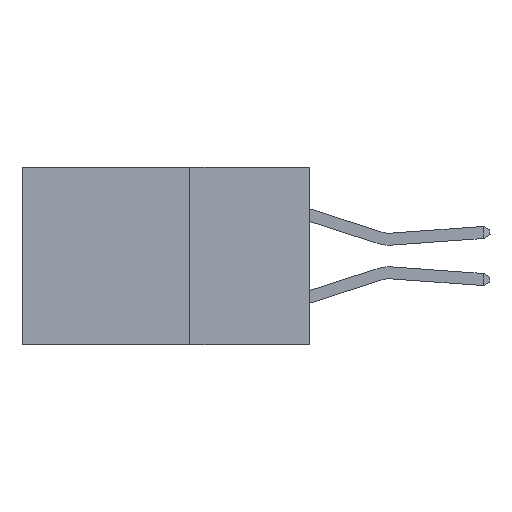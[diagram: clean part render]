
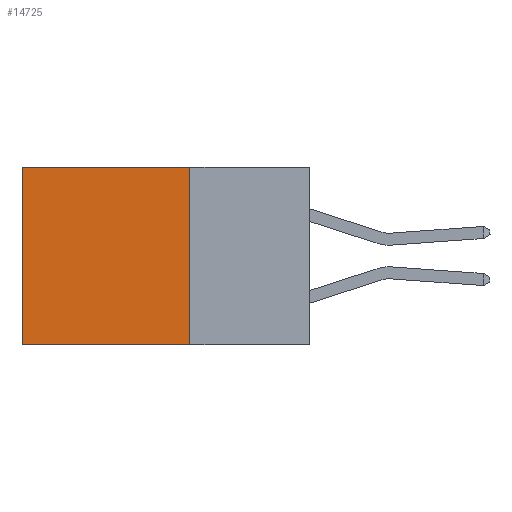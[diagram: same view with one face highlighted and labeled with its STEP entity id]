
A CAD part, left-side view. The second image highlights one B-rep face of the part: STEP entity #14725.
In plain terms, the highlighted planar face has unit normal (-1, 0, 0).
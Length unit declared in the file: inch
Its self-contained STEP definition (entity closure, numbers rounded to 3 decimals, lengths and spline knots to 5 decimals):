
#512 = VERTEX_POINT ( 'NONE', #18626 ) ;
#683 = EDGE_CURVE ( 'NONE', #512, #9621, #8104, .T. ) ;
#892 = CARTESIAN_POINT ( 'NONE',  ( 0.2615, 0.25, -0.37 ) ) ;
#1943 = EDGE_CURVE ( 'NONE', #512, #4244, #17350, .T. ) ;
#2690 = DIRECTION ( 'NONE',  ( 0., 0., -1. ) ) ;
#2937 = AXIS2_PLACEMENT_3D ( 'NONE', #4848, #11272, #3156 ) ;
#3156 = DIRECTION ( 'NONE',  ( 0., 0., -1. ) ) ;
#3219 = DIRECTION ( 'NONE',  ( 0., 1., 0. ) ) ;
#3488 = DIRECTION ( 'NONE',  ( 0., 0., -1. ) ) ;
#4244 = VERTEX_POINT ( 'NONE', #7493 ) ;
#4326 = CARTESIAN_POINT ( 'NONE',  ( 0.2615, 0.6, -0.37 ) ) ;
#4394 = CARTESIAN_POINT ( 'NONE',  ( 0.2615, 0.25, 0. ) ) ;
#4531 = DIRECTION ( 'NONE',  ( 0., 1., 0. ) ) ;
#4848 = CARTESIAN_POINT ( 'NONE',  ( 0.2615, 0.25, -0.37 ) ) ;
#6110 = CARTESIAN_POINT ( 'NONE',  ( 0.2615, 0.6, 0. ) ) ;
#6906 = VERTEX_POINT ( 'NONE', #4326 ) ;
#7493 = CARTESIAN_POINT ( 'NONE',  ( 0.2615, 0.25, -0.37 ) ) ;
#8104 = LINE ( 'NONE', #4394, #9798 ) ;
#9035 = EDGE_CURVE ( 'NONE', #9621, #6906, #11935, .T. ) ;
#9621 = VERTEX_POINT ( 'NONE', #6110 ) ;
#9798 = VECTOR ( 'NONE', #3219, 39.37008 ) ;
#10248 = ORIENTED_EDGE ( 'NONE', *, *, #683, .T. ) ;
#10305 = EDGE_LOOP ( 'NONE', ( #15643, #13371, #19847, #10248 ) ) ;
#10400 = VECTOR ( 'NONE', #4531, 39.37008 ) ;
#11272 = DIRECTION ( 'NONE',  ( 1., 0., 0. ) ) ;
#11533 = EDGE_CURVE ( 'NONE', #4244, #6906, #20800, .T. ) ;
#11935 = LINE ( 'NONE', #18462, #13082 ) ;
#13082 = VECTOR ( 'NONE', #3488, 39.37008 ) ;
#13371 = ORIENTED_EDGE ( 'NONE', *, *, #11533, .F. ) ;
#14725 = ADVANCED_FACE ( 'NONE', ( #15900 ), #17915, .F. ) ;
#15643 = ORIENTED_EDGE ( 'NONE', *, *, #9035, .T. ) ;
#15900 = FACE_OUTER_BOUND ( 'NONE', #10305, .T. ) ;
#17350 = LINE ( 'NONE', #892, #20774 ) ;
#17386 = CARTESIAN_POINT ( 'NONE',  ( 0.2615, 0.25, -0.37 ) ) ;
#17915 = PLANE ( 'NONE',  #2937 ) ;
#18462 = CARTESIAN_POINT ( 'NONE',  ( 0.2615, 0.6, -0.37 ) ) ;
#18626 = CARTESIAN_POINT ( 'NONE',  ( 0.2615, 0.25, 0. ) ) ;
#19847 = ORIENTED_EDGE ( 'NONE', *, *, #1943, .F. ) ;
#20774 = VECTOR ( 'NONE', #2690, 39.37008 ) ;
#20800 = LINE ( 'NONE', #17386, #10400 ) ;
